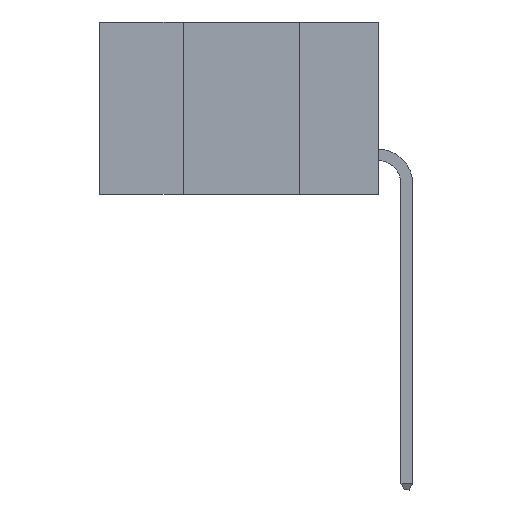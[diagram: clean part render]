
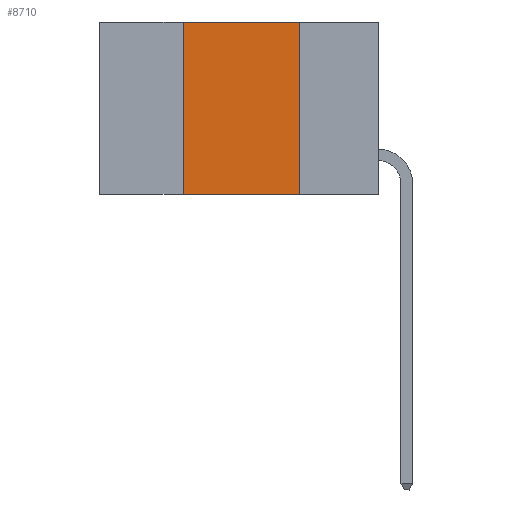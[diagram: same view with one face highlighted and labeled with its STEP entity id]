
A CAD part, left-side view. The second image highlights one B-rep face of the part: STEP entity #8710.
In plain terms, the highlighted planar face has unit normal (-1, 0, 0).
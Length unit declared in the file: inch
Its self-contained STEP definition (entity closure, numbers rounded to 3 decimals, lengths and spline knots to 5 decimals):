
#346 = CARTESIAN_POINT ( 'NONE',  ( 0., 0.42, 0. ) ) ;
#1100 = DIRECTION ( 'NONE',  ( 0., 0., 1. ) ) ;
#1633 = VECTOR ( 'NONE', #10752, 39.37008 ) ;
#1751 = VECTOR ( 'NONE', #5552, 39.37008 ) ;
#1865 = ORIENTED_EDGE ( 'NONE', *, *, #2319, .T. ) ;
#1959 = CARTESIAN_POINT ( 'NONE',  ( 0., 0.17, 0. ) ) ;
#2319 = EDGE_CURVE ( 'NONE', #6689, #10202, #5270, .T. ) ;
#2378 = CARTESIAN_POINT ( 'NONE',  ( 0., 0.6, 0. ) ) ;
#2579 = EDGE_CURVE ( 'NONE', #4836, #4330, #5544, .T. ) ;
#2939 = CARTESIAN_POINT ( 'NONE',  ( 0., 0.6, -0.37 ) ) ;
#2999 = CARTESIAN_POINT ( 'NONE',  ( 0., 0.17, 0. ) ) ;
#3539 = LINE ( 'NONE', #5179, #8297 ) ;
#4330 = VERTEX_POINT ( 'NONE', #1959 ) ;
#4402 = ORIENTED_EDGE ( 'NONE', *, *, #8632, .F. ) ;
#4836 = VERTEX_POINT ( 'NONE', #346 ) ;
#4954 = DIRECTION ( 'NONE',  ( 1., 0., 0. ) ) ;
#5179 = CARTESIAN_POINT ( 'NONE',  ( 0., 0.42, 0. ) ) ;
#5270 = LINE ( 'NONE', #2939, #1751 ) ;
#5544 = LINE ( 'NONE', #7149, #1633 ) ;
#5552 = DIRECTION ( 'NONE',  ( 0., -1., 0. ) ) ;
#5661 = CARTESIAN_POINT ( 'NONE',  ( 0., 0.42, -0.37 ) ) ;
#6689 = VERTEX_POINT ( 'NONE', #5661 ) ;
#6721 = ORIENTED_EDGE ( 'NONE', *, *, #2579, .F. ) ;
#6808 = VECTOR ( 'NONE', #9001, 39.37008 ) ;
#7144 = ORIENTED_EDGE ( 'NONE', *, *, #9491, .F. ) ;
#7149 = CARTESIAN_POINT ( 'NONE',  ( 0., 0.6, 0. ) ) ;
#8297 = VECTOR ( 'NONE', #1100, 39.37008 ) ;
#8577 = CARTESIAN_POINT ( 'NONE',  ( 0., 0.17, -0.37 ) ) ;
#8631 = EDGE_LOOP ( 'NONE', ( #4402, #6721, #7144, #1865 ) ) ;
#8632 = EDGE_CURVE ( 'NONE', #4330, #10202, #9406, .T. ) ;
#8710 = ADVANCED_FACE ( 'NONE', ( #11040 ), #10150, .F. ) ;
#9001 = DIRECTION ( 'NONE',  ( 0., 0., -1. ) ) ;
#9406 = LINE ( 'NONE', #2999, #6808 ) ;
#9491 = EDGE_CURVE ( 'NONE', #6689, #4836, #3539, .T. ) ;
#10021 = AXIS2_PLACEMENT_3D ( 'NONE', #2378, #4954, #10860 ) ;
#10150 = PLANE ( 'NONE',  #10021 ) ;
#10202 = VERTEX_POINT ( 'NONE', #8577 ) ;
#10752 = DIRECTION ( 'NONE',  ( 0., -1., 0. ) ) ;
#10860 = DIRECTION ( 'NONE',  ( 0., 0., -1. ) ) ;
#11040 = FACE_OUTER_BOUND ( 'NONE', #8631, .T. ) ;
